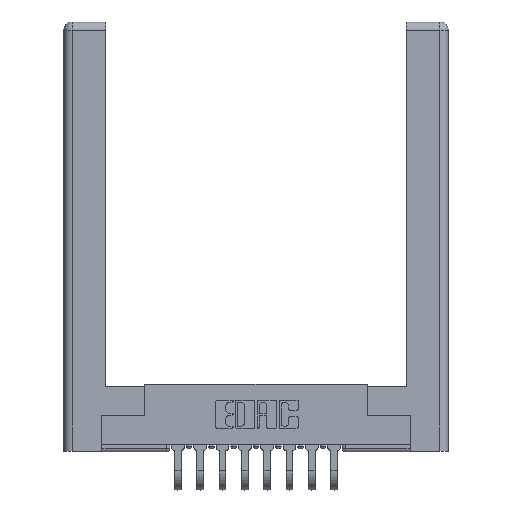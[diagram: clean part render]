
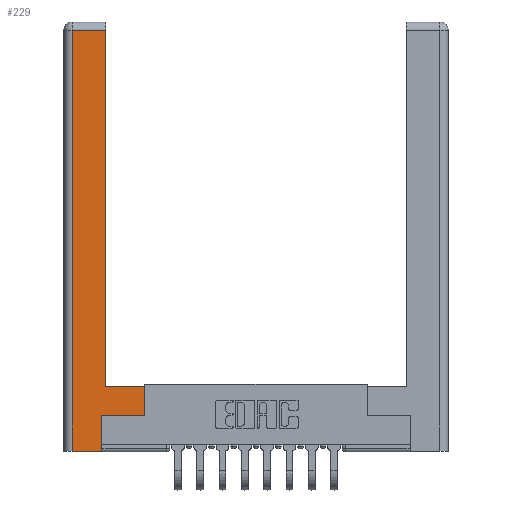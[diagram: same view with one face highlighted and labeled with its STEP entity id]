
A CAD part, top view. The second image highlights one B-rep face of the part: STEP entity #229.
In plain terms, the highlighted planar face has unit normal (0, 0, 1).
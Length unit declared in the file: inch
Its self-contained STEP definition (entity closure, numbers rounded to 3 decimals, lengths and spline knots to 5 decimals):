
#229 = ADVANCED_FACE ( 'NONE', ( #8311 ), #8097, .F. ) ;
#681 = DIRECTION ( 'NONE',  ( 0., 0., -1. ) ) ;
#758 = CARTESIAN_POINT ( 'NONE',  ( 0.565, 0.245, 0. ) ) ;
#991 = LINE ( 'NONE', #758, #6947 ) ;
#1436 = CARTESIAN_POINT ( 'NONE',  ( 0.265, 0., 0. ) ) ;
#1707 = VECTOR ( 'NONE', #4731, 39.37008 ) ;
#1715 = LINE ( 'NONE', #8875, #1707 ) ;
#1889 = VERTEX_POINT ( 'NONE', #1436 ) ;
#1947 = LINE ( 'NONE', #13671, #3290 ) ;
#1997 = AXIS2_PLACEMENT_3D ( 'NONE', #2961, #681, #7193 ) ;
#2036 = ORIENTED_EDGE ( 'NONE', *, *, #3512, .T. ) ;
#2248 = EDGE_CURVE ( 'NONE', #2382, #2790, #3674, .T. ) ;
#2382 = VERTEX_POINT ( 'NONE', #3752 ) ;
#2516 = ORIENTED_EDGE ( 'NONE', *, *, #11833, .T. ) ;
#2567 = EDGE_CURVE ( 'NONE', #12894, #2382, #991, .T. ) ;
#2576 = VECTOR ( 'NONE', #9701, 39.37008 ) ;
#2725 = ORIENTED_EDGE ( 'NONE', *, *, #4557, .T. ) ;
#2790 = VERTEX_POINT ( 'NONE', #8566 ) ;
#2961 = CARTESIAN_POINT ( 'NONE',  ( 0., 0., 0. ) ) ;
#3290 = VECTOR ( 'NONE', #7519, 39.37008 ) ;
#3512 = EDGE_CURVE ( 'NONE', #11596, #1889, #8963, .T. ) ;
#3569 = DIRECTION ( 'NONE',  ( 1., 0., 0. ) ) ;
#3674 = LINE ( 'NONE', #4518, #7386 ) ;
#3752 = CARTESIAN_POINT ( 'NONE',  ( 0.565, 0.245, 0. ) ) ;
#4009 = ORIENTED_EDGE ( 'NONE', *, *, #11417, .T. ) ;
#4347 = CARTESIAN_POINT ( 'NONE',  ( 0.295, 0.45, 0. ) ) ;
#4518 = CARTESIAN_POINT ( 'NONE',  ( 0.565, 0.45, 0. ) ) ;
#4557 = EDGE_CURVE ( 'NONE', #11539, #9418, #7400, .T. ) ;
#4693 = VECTOR ( 'NONE', #10721, 39.37008 ) ;
#4731 = DIRECTION ( 'NONE',  ( 0., 1., 0. ) ) ;
#5342 = CARTESIAN_POINT ( 'NONE',  ( 0.265, 0.245, 0. ) ) ;
#5498 = VECTOR ( 'NONE', #5622, 39.37008 ) ;
#5622 = DIRECTION ( 'NONE',  ( 0., -1., 0. ) ) ;
#6436 = CARTESIAN_POINT ( 'NONE',  ( 0.295, 3., 0. ) ) ;
#6821 = CARTESIAN_POINT ( 'NONE',  ( 0.265, 0., 0. ) ) ;
#6846 = CARTESIAN_POINT ( 'NONE',  ( 0.295, 2.94, 0. ) ) ;
#6947 = VECTOR ( 'NONE', #8506, 39.37008 ) ;
#7193 = DIRECTION ( 'NONE',  ( -1., 0., 0. ) ) ;
#7300 = CARTESIAN_POINT ( 'NONE',  ( 0.0615, 0., 0. ) ) ;
#7386 = VECTOR ( 'NONE', #7886, 39.37008 ) ;
#7400 = LINE ( 'NONE', #6436, #4693 ) ;
#7409 = LINE ( 'NONE', #7538, #2576 ) ;
#7519 = DIRECTION ( 'NONE',  ( -1., 0., 0. ) ) ;
#7538 = CARTESIAN_POINT ( 'NONE',  ( 0.0615, 2.94, 0. ) ) ;
#7741 = ORIENTED_EDGE ( 'NONE', *, *, #10551, .T. ) ;
#7886 = DIRECTION ( 'NONE',  ( 0., 1., 0. ) ) ;
#8071 = CARTESIAN_POINT ( 'NONE',  ( 0.0615, 2.94, 0. ) ) ;
#8097 = PLANE ( 'NONE',  #1997 ) ;
#8311 = FACE_OUTER_BOUND ( 'NONE', #10650, .T. ) ;
#8506 = DIRECTION ( 'NONE',  ( 1., 0., 0. ) ) ;
#8566 = CARTESIAN_POINT ( 'NONE',  ( 0.565, 0.45, 0. ) ) ;
#8734 = CARTESIAN_POINT ( 'NONE',  ( 0.0615, 0., 0. ) ) ;
#8765 = EDGE_CURVE ( 'NONE', #9418, #9949, #7409, .T. ) ;
#8786 = ORIENTED_EDGE ( 'NONE', *, *, #2567, .T. ) ;
#8875 = CARTESIAN_POINT ( 'NONE',  ( 0.265, 0.245, 0. ) ) ;
#8963 = LINE ( 'NONE', #6821, #11875 ) ;
#9418 = VERTEX_POINT ( 'NONE', #6846 ) ;
#9701 = DIRECTION ( 'NONE',  ( -1., 0., 0. ) ) ;
#9949 = VERTEX_POINT ( 'NONE', #8071 ) ;
#10551 = EDGE_CURVE ( 'NONE', #9949, #11596, #13211, .T. ) ;
#10650 = EDGE_LOOP ( 'NONE', ( #2725, #11384, #7741, #2036, #2516, #8786, #11019, #4009 ) ) ;
#10721 = DIRECTION ( 'NONE',  ( 0., 1., 0. ) ) ;
#11019 = ORIENTED_EDGE ( 'NONE', *, *, #2248, .T. ) ;
#11384 = ORIENTED_EDGE ( 'NONE', *, *, #8765, .T. ) ;
#11417 = EDGE_CURVE ( 'NONE', #2790, #11539, #1947, .T. ) ;
#11539 = VERTEX_POINT ( 'NONE', #4347 ) ;
#11596 = VERTEX_POINT ( 'NONE', #7300 ) ;
#11833 = EDGE_CURVE ( 'NONE', #1889, #12894, #1715, .T. ) ;
#11875 = VECTOR ( 'NONE', #3569, 39.37008 ) ;
#12894 = VERTEX_POINT ( 'NONE', #5342 ) ;
#13211 = LINE ( 'NONE', #8734, #5498 ) ;
#13671 = CARTESIAN_POINT ( 'NONE',  ( 0.295, 0.45, 0. ) ) ;
